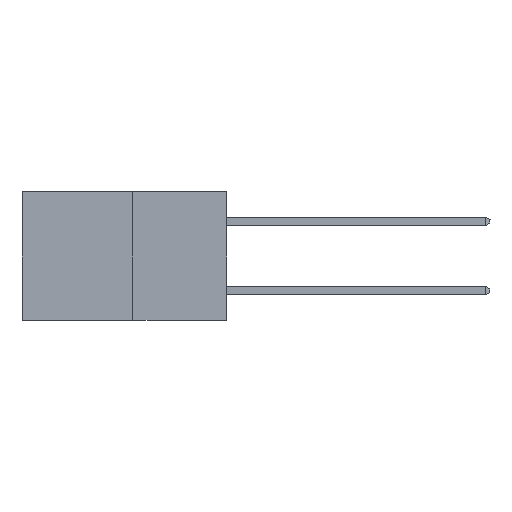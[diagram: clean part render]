
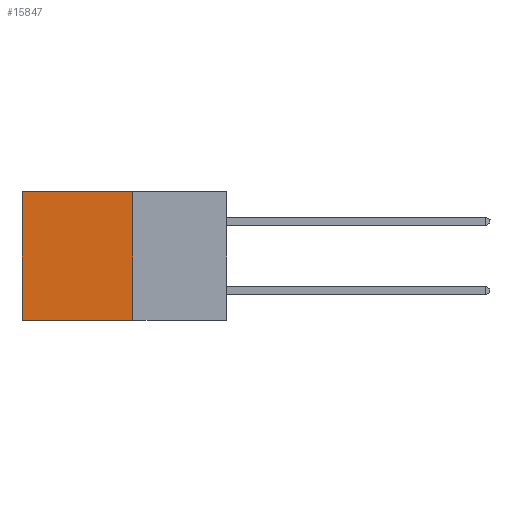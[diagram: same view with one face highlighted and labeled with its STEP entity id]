
A CAD part, left-side view. The second image highlights one B-rep face of the part: STEP entity #15847.
In plain terms, the highlighted planar face has unit normal (-1, 0, 0).
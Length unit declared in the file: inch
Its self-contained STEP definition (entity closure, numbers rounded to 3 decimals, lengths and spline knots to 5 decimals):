
#38 = DIRECTION ( 'NONE',  ( 0., 0., -1. ) ) ;
#130 = AXIS2_PLACEMENT_3D ( 'NONE', #11471, #13583, #1019 ) ;
#1019 = DIRECTION ( 'NONE',  ( 0., 0., -1. ) ) ;
#1262 = VECTOR ( 'NONE', #15902, 39.37008 ) ;
#2347 = LINE ( 'NONE', #25712, #12810 ) ;
#3863 = VERTEX_POINT ( 'NONE', #19283 ) ;
#4115 = ORIENTED_EDGE ( 'NONE', *, *, #5433, .F. ) ;
#5049 = CARTESIAN_POINT ( 'NONE',  ( 0.277, 0.27, -0.37 ) ) ;
#5433 = EDGE_CURVE ( 'NONE', #3863, #24109, #2347, .T. ) ;
#5552 = CARTESIAN_POINT ( 'NONE',  ( 0.277, 0.27, 0. ) ) ;
#6291 = CARTESIAN_POINT ( 'NONE',  ( 0.277, 0.59, -0.37 ) ) ;
#6561 = ORIENTED_EDGE ( 'NONE', *, *, #14186, .T. ) ;
#6662 = ORIENTED_EDGE ( 'NONE', *, *, #16683, .T. ) ;
#7456 = VERTEX_POINT ( 'NONE', #18183 ) ;
#10107 = FACE_OUTER_BOUND ( 'NONE', #16657, .T. ) ;
#11471 = CARTESIAN_POINT ( 'NONE',  ( 0.277, 0.27, -0.37 ) ) ;
#12176 = EDGE_CURVE ( 'NONE', #24109, #7456, #19208, .T. ) ;
#12810 = VECTOR ( 'NONE', #38, 39.37008 ) ;
#13583 = DIRECTION ( 'NONE',  ( 1., 0., 0. ) ) ;
#13752 = VECTOR ( 'NONE', #18766, 39.37008 ) ;
#14186 = EDGE_CURVE ( 'NONE', #24948, #7456, #20711, .T. ) ;
#15847 = ADVANCED_FACE ( 'NONE', ( #10107 ), #23861, .F. ) ;
#15902 = DIRECTION ( 'NONE',  ( 0., 1., 0. ) ) ;
#16657 = EDGE_LOOP ( 'NONE', ( #6561, #24231, #4115, #6662 ) ) ;
#16683 = EDGE_CURVE ( 'NONE', #3863, #24948, #22730, .T. ) ;
#18183 = CARTESIAN_POINT ( 'NONE',  ( 0.277, 0.59, -0.37 ) ) ;
#18766 = DIRECTION ( 'NONE',  ( 0., 1., 0. ) ) ;
#19208 = LINE ( 'NONE', #22832, #13752 ) ;
#19283 = CARTESIAN_POINT ( 'NONE',  ( 0.277, 0.27, 0. ) ) ;
#20711 = LINE ( 'NONE', #6291, #25577 ) ;
#22730 = LINE ( 'NONE', #5552, #1262 ) ;
#22832 = CARTESIAN_POINT ( 'NONE',  ( 0.277, 0.27, -0.37 ) ) ;
#22838 = DIRECTION ( 'NONE',  ( 0., 0., -1. ) ) ;
#23861 = PLANE ( 'NONE',  #130 ) ;
#24109 = VERTEX_POINT ( 'NONE', #5049 ) ;
#24231 = ORIENTED_EDGE ( 'NONE', *, *, #12176, .F. ) ;
#24948 = VERTEX_POINT ( 'NONE', #26185 ) ;
#25577 = VECTOR ( 'NONE', #22838, 39.37008 ) ;
#25712 = CARTESIAN_POINT ( 'NONE',  ( 0.277, 0.27, -0.37 ) ) ;
#26185 = CARTESIAN_POINT ( 'NONE',  ( 0.277, 0.59, 0. ) ) ;
